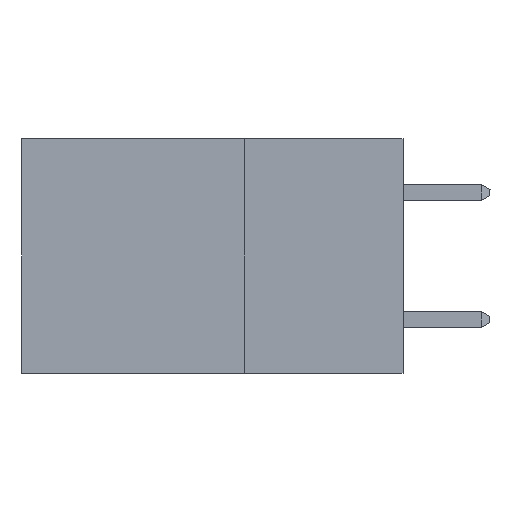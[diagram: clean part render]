
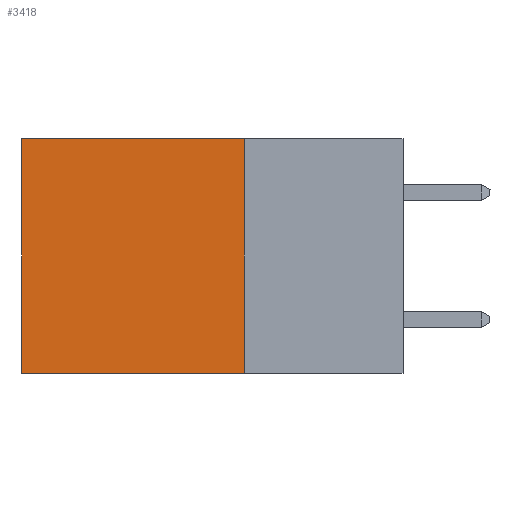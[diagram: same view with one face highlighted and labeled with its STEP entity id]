
A CAD part, left-side view. The second image highlights one B-rep face of the part: STEP entity #3418.
In plain terms, the highlighted planar face has unit normal (-1, 0, 0).
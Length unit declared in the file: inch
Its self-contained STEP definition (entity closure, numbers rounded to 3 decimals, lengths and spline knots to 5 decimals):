
#304 = CARTESIAN_POINT ( 'NONE',  ( 0.2875, 0.25, -0.37 ) ) ;
#827 = ORIENTED_EDGE ( 'NONE', *, *, #9553, .T. ) ;
#2020 = EDGE_LOOP ( 'NONE', ( #827, #15751, #2656, #20949 ) ) ;
#2626 = DIRECTION ( 'NONE',  ( 0., 1., 0. ) ) ;
#2656 = ORIENTED_EDGE ( 'NONE', *, *, #13609, .F. ) ;
#3291 = DIRECTION ( 'NONE',  ( 0., 0., -1. ) ) ;
#3418 = ADVANCED_FACE ( 'NONE', ( #7651 ), #4445, .F. ) ;
#3714 = VECTOR ( 'NONE', #2626, 39.37008 ) ;
#4445 = PLANE ( 'NONE',  #16233 ) ;
#5049 = CARTESIAN_POINT ( 'NONE',  ( 0.2875, 0.6, -0.37 ) ) ;
#5360 = LINE ( 'NONE', #10205, #14137 ) ;
#5776 = VERTEX_POINT ( 'NONE', #6802 ) ;
#6148 = DIRECTION ( 'NONE',  ( 0., 0., -1. ) ) ;
#6802 = CARTESIAN_POINT ( 'NONE',  ( 0.2875, 0.25, 0. ) ) ;
#7236 = DIRECTION ( 'NONE',  ( 0., 1., 0. ) ) ;
#7651 = FACE_OUTER_BOUND ( 'NONE', #2020, .T. ) ;
#9553 = EDGE_CURVE ( 'NONE', #17576, #12951, #15250, .T. ) ;
#10205 = CARTESIAN_POINT ( 'NONE',  ( 0.2875, 0.25, 0. ) ) ;
#10423 = VECTOR ( 'NONE', #7236, 39.37008 ) ;
#10529 = VECTOR ( 'NONE', #17039, 39.37008 ) ;
#11363 = CARTESIAN_POINT ( 'NONE',  ( 0.2875, 0.25, 0. ) ) ;
#11364 = CARTESIAN_POINT ( 'NONE',  ( 0.2875, 0.25, 0. ) ) ;
#11647 = CARTESIAN_POINT ( 'NONE',  ( 0.2875, 0.6, 0. ) ) ;
#12684 = CARTESIAN_POINT ( 'NONE',  ( 0.2875, 0.25, -0.37 ) ) ;
#12951 = VERTEX_POINT ( 'NONE', #5049 ) ;
#13609 = EDGE_CURVE ( 'NONE', #5776, #21363, #5360, .T. ) ;
#14137 = VECTOR ( 'NONE', #3291, 39.37008 ) ;
#15250 = LINE ( 'NONE', #11647, #10529 ) ;
#15672 = LINE ( 'NONE', #304, #10423 ) ;
#15751 = ORIENTED_EDGE ( 'NONE', *, *, #21316, .F. ) ;
#15988 = CARTESIAN_POINT ( 'NONE',  ( 0.2875, 0.6, 0. ) ) ;
#16233 = AXIS2_PLACEMENT_3D ( 'NONE', #11364, #16689, #6148 ) ;
#16689 = DIRECTION ( 'NONE',  ( 1., 0., 0. ) ) ;
#17039 = DIRECTION ( 'NONE',  ( 0., 0., -1. ) ) ;
#17576 = VERTEX_POINT ( 'NONE', #15988 ) ;
#19688 = EDGE_CURVE ( 'NONE', #5776, #17576, #22141, .T. ) ;
#20949 = ORIENTED_EDGE ( 'NONE', *, *, #19688, .T. ) ;
#21316 = EDGE_CURVE ( 'NONE', #21363, #12951, #15672, .T. ) ;
#21363 = VERTEX_POINT ( 'NONE', #12684 ) ;
#22141 = LINE ( 'NONE', #11363, #3714 ) ;
